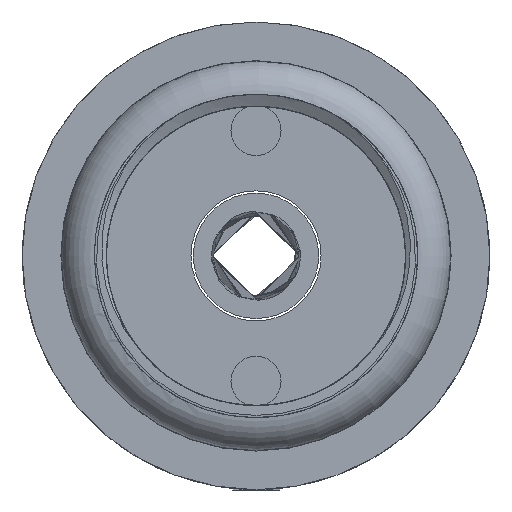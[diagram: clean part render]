
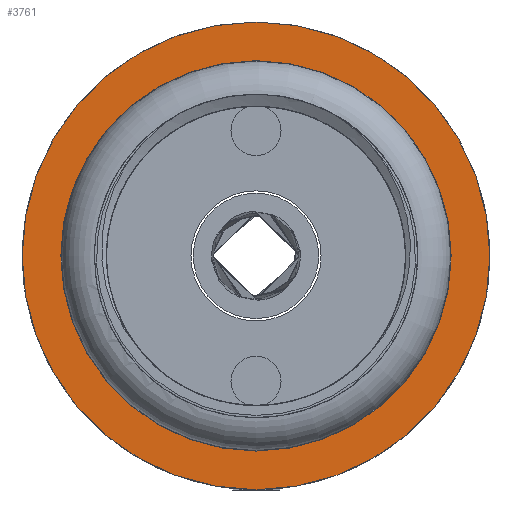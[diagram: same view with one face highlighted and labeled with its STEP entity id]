
A CAD part, left-side view. The second image highlights one B-rep face of the part: STEP entity #3761.
In plain terms, the highlighted planar face has unit normal (-1, 0, 0).
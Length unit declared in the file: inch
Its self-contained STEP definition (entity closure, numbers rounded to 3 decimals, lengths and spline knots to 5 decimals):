
#467=FACE_BOUND('',#918,.T.);
#487=PLANE('',#3990);
#678=FACE_OUTER_BOUND('',#917,.T.);
#917=EDGE_LOOP('',(#3280));
#918=EDGE_LOOP('',(#3281));
#1375=CIRCLE('',#3991,0.5875);
#1376=CIRCLE('',#3992,0.49025);
#1710=VERTEX_POINT('',#18669);
#1711=VERTEX_POINT('',#18671);
#2247=EDGE_CURVE('',#1710,#1710,#1375,.T.);
#2248=EDGE_CURVE('',#1711,#1711,#1376,.T.);
#3280=ORIENTED_EDGE('',*,*,#2247,.T.);
#3281=ORIENTED_EDGE('',*,*,#2248,.F.);
#3761=ADVANCED_FACE('',(#678,#467),#487,.T.);
#3990=AXIS2_PLACEMENT_3D('',#18668,#4510,#4511);
#3991=AXIS2_PLACEMENT_3D('',#18670,#4512,#4513);
#3992=AXIS2_PLACEMENT_3D('',#18672,#4514,#4515);
#4510=DIRECTION('center_axis',(-1.,0.,0.));
#4511=DIRECTION('ref_axis',(0.,0.,1.));
#4512=DIRECTION('center_axis',(-1.,0.,0.));
#4513=DIRECTION('ref_axis',(0.,0.,1.));
#4514=DIRECTION('center_axis',(-1.,0.,0.));
#4515=DIRECTION('ref_axis',(0.,-1.,0.));
#18668=CARTESIAN_POINT('Origin',(-4.60501,0.96279,0.21529));
#18669=CARTESIAN_POINT('',(-4.60501,0.96279,0.80279));
#18670=CARTESIAN_POINT('Origin',(-4.60501,0.96279,0.21529));
#18671=CARTESIAN_POINT('',(-4.60501,1.45304,0.21529));
#18672=CARTESIAN_POINT('Origin',(-4.60501,0.96279,0.21529));
